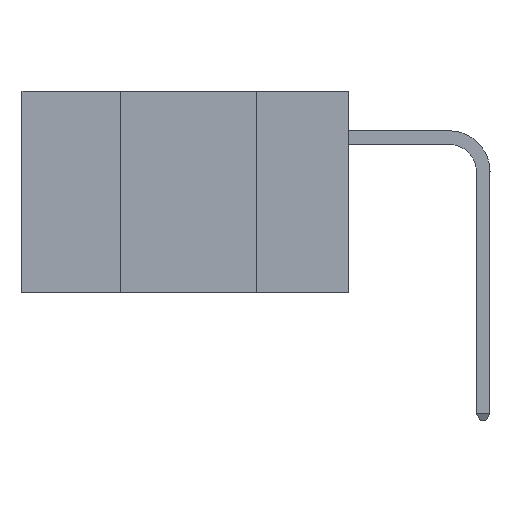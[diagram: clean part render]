
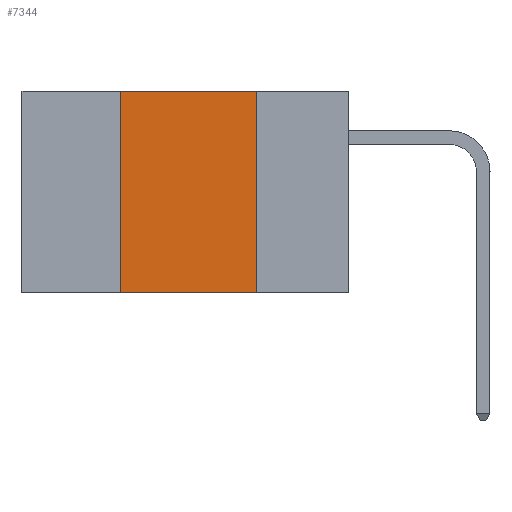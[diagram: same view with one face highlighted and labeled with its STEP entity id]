
A CAD part, left-side view. The second image highlights one B-rep face of the part: STEP entity #7344.
In plain terms, the highlighted planar face has unit normal (-1, 0, 0).
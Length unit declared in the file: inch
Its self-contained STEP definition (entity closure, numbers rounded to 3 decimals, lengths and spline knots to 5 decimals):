
#224 = LINE ( 'NONE', #2497, #8346 ) ;
#949 = LINE ( 'NONE', #15143, #9057 ) ;
#1600 = ORIENTED_EDGE ( 'NONE', *, *, #10104, .F. ) ;
#1739 = ORIENTED_EDGE ( 'NONE', *, *, #3092, .F. ) ;
#1756 = ORIENTED_EDGE ( 'NONE', *, *, #9048, .F. ) ;
#1793 = ORIENTED_EDGE ( 'NONE', *, *, #5889, .T. ) ;
#2436 = VERTEX_POINT ( 'NONE', #16426 ) ;
#2497 = CARTESIAN_POINT ( 'NONE',  ( 0., 0.17, 0. ) ) ;
#2528 = PLANE ( 'NONE',  #8533 ) ;
#3092 = EDGE_CURVE ( 'NONE', #19693, #12035, #19698, .T. ) ;
#4269 = CARTESIAN_POINT ( 'NONE',  ( 0., 0.42, -0.37 ) ) ;
#5052 = EDGE_LOOP ( 'NONE', ( #1600, #1739, #1756, #1793 ) ) ;
#5889 = EDGE_CURVE ( 'NONE', #9438, #2436, #949, .T. ) ;
#6747 = LINE ( 'NONE', #15762, #14353 ) ;
#7344 = ADVANCED_FACE ( 'NONE', ( #12312 ), #2528, .F. ) ;
#7698 = DIRECTION ( 'NONE',  ( 0., -1., 0. ) ) ;
#8346 = VECTOR ( 'NONE', #19463, 39.37008 ) ;
#8533 = AXIS2_PLACEMENT_3D ( 'NONE', #16528, #9047, #19492 ) ;
#9047 = DIRECTION ( 'NONE',  ( 1., 0., 0. ) ) ;
#9048 = EDGE_CURVE ( 'NONE', #9438, #19693, #6747, .T. ) ;
#9057 = VECTOR ( 'NONE', #7698, 39.37008 ) ;
#9438 = VERTEX_POINT ( 'NONE', #4269 ) ;
#10104 = EDGE_CURVE ( 'NONE', #12035, #2436, #224, .T. ) ;
#11824 = VECTOR ( 'NONE', #13689, 39.37008 ) ;
#12035 = VERTEX_POINT ( 'NONE', #18778 ) ;
#12210 = CARTESIAN_POINT ( 'NONE',  ( 0., 0.6, 0. ) ) ;
#12312 = FACE_OUTER_BOUND ( 'NONE', #5052, .T. ) ;
#13689 = DIRECTION ( 'NONE',  ( 0., -1., 0. ) ) ;
#14167 = CARTESIAN_POINT ( 'NONE',  ( 0., 0.42, 0. ) ) ;
#14353 = VECTOR ( 'NONE', #18745, 39.37008 ) ;
#15143 = CARTESIAN_POINT ( 'NONE',  ( 0., 0.6, -0.37 ) ) ;
#15762 = CARTESIAN_POINT ( 'NONE',  ( 0., 0.42, 0. ) ) ;
#16426 = CARTESIAN_POINT ( 'NONE',  ( 0., 0.17, -0.37 ) ) ;
#16528 = CARTESIAN_POINT ( 'NONE',  ( 0., 0.6, 0. ) ) ;
#18745 = DIRECTION ( 'NONE',  ( 0., 0., 1. ) ) ;
#18778 = CARTESIAN_POINT ( 'NONE',  ( 0., 0.17, 0. ) ) ;
#19463 = DIRECTION ( 'NONE',  ( 0., 0., -1. ) ) ;
#19492 = DIRECTION ( 'NONE',  ( 0., 0., -1. ) ) ;
#19693 = VERTEX_POINT ( 'NONE', #14167 ) ;
#19698 = LINE ( 'NONE', #12210, #11824 ) ;
